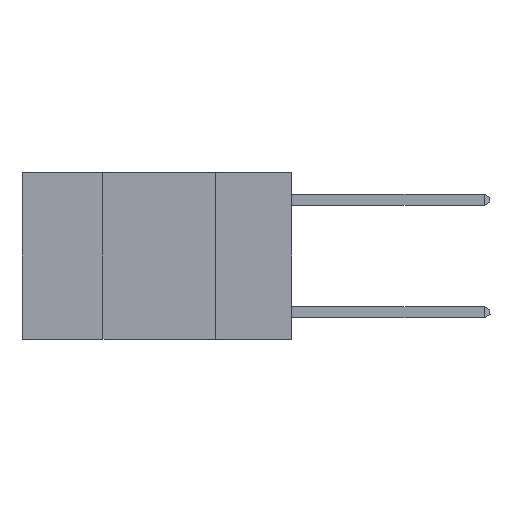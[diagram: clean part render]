
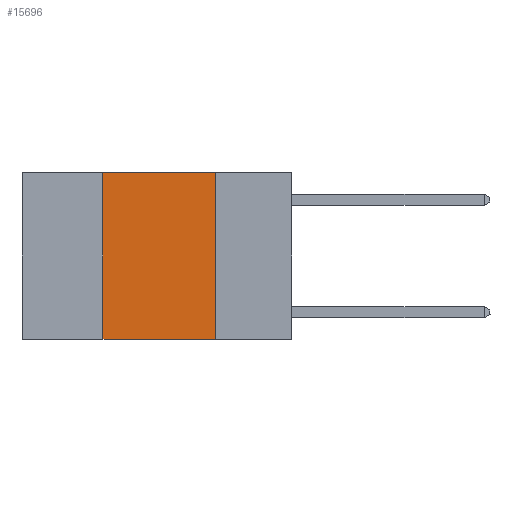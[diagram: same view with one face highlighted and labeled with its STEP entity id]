
A CAD part, left-side view. The second image highlights one B-rep face of the part: STEP entity #15696.
In plain terms, the highlighted planar face has unit normal (-1, 0, 0).
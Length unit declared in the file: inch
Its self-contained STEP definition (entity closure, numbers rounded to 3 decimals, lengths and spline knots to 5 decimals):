
#778 = CARTESIAN_POINT ( 'NONE',  ( 0., 0.42, -0.37 ) ) ;
#2139 = VECTOR ( 'NONE', #2441, 39.37008 ) ;
#2351 = ORIENTED_EDGE ( 'NONE', *, *, #4697, .F. ) ;
#2379 = CARTESIAN_POINT ( 'NONE',  ( 0., 0.6, -0.37 ) ) ;
#2441 = DIRECTION ( 'NONE',  ( 0., -1., 0. ) ) ;
#3069 = EDGE_LOOP ( 'NONE', ( #6056, #13457, #2351, #4628 ) ) ;
#3764 = DIRECTION ( 'NONE',  ( 0., -1., 0. ) ) ;
#4628 = ORIENTED_EDGE ( 'NONE', *, *, #4796, .T. ) ;
#4697 = EDGE_CURVE ( 'NONE', #15226, #11327, #17195, .T. ) ;
#4796 = EDGE_CURVE ( 'NONE', #15226, #12525, #16370, .T. ) ;
#4950 = EDGE_CURVE ( 'NONE', #11327, #12888, #6804, .T. ) ;
#5080 = DIRECTION ( 'NONE',  ( 0., 0., -1. ) ) ;
#5144 = CARTESIAN_POINT ( 'NONE',  ( 0., 0.17, 0. ) ) ;
#5970 = CARTESIAN_POINT ( 'NONE',  ( 0., 0.42, 0. ) ) ;
#6056 = ORIENTED_EDGE ( 'NONE', *, *, #7605, .F. ) ;
#6100 = DIRECTION ( 'NONE',  ( 1., 0., 0. ) ) ;
#6187 = PLANE ( 'NONE',  #7600 ) ;
#6804 = LINE ( 'NONE', #16820, #2139 ) ;
#7600 = AXIS2_PLACEMENT_3D ( 'NONE', #12077, #6100, #5080 ) ;
#7605 = EDGE_CURVE ( 'NONE', #12888, #12525, #16907, .T. ) ;
#7849 = FACE_OUTER_BOUND ( 'NONE', #3069, .T. ) ;
#9274 = VECTOR ( 'NONE', #11301, 39.37008 ) ;
#9313 = CARTESIAN_POINT ( 'NONE',  ( 0., 0.17, -0.37 ) ) ;
#11301 = DIRECTION ( 'NONE',  ( 0., 0., -1. ) ) ;
#11327 = VERTEX_POINT ( 'NONE', #14580 ) ;
#12077 = CARTESIAN_POINT ( 'NONE',  ( 0., 0.6, 0. ) ) ;
#12525 = VERTEX_POINT ( 'NONE', #9313 ) ;
#12888 = VERTEX_POINT ( 'NONE', #5144 ) ;
#13457 = ORIENTED_EDGE ( 'NONE', *, *, #4950, .F. ) ;
#13788 = CARTESIAN_POINT ( 'NONE',  ( 0., 0.17, 0. ) ) ;
#13888 = VECTOR ( 'NONE', #3764, 39.37008 ) ;
#14580 = CARTESIAN_POINT ( 'NONE',  ( 0., 0.42, 0. ) ) ;
#15226 = VERTEX_POINT ( 'NONE', #778 ) ;
#15696 = ADVANCED_FACE ( 'NONE', ( #7849 ), #6187, .F. ) ;
#15993 = DIRECTION ( 'NONE',  ( 0., 0., 1. ) ) ;
#16370 = LINE ( 'NONE', #2379, #13888 ) ;
#16538 = VECTOR ( 'NONE', #15993, 39.37008 ) ;
#16820 = CARTESIAN_POINT ( 'NONE',  ( 0., 0.6, 0. ) ) ;
#16907 = LINE ( 'NONE', #13788, #9274 ) ;
#17195 = LINE ( 'NONE', #5970, #16538 ) ;
